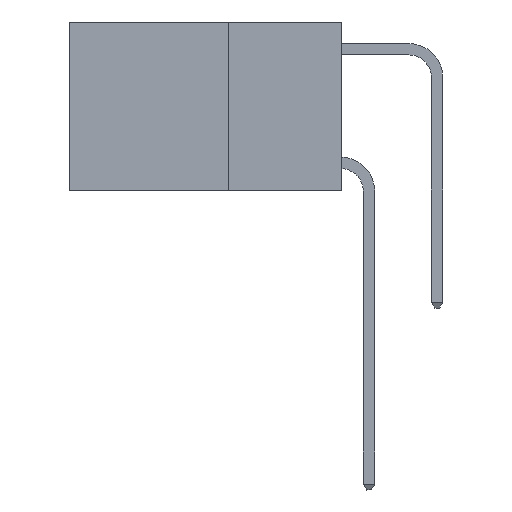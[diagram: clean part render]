
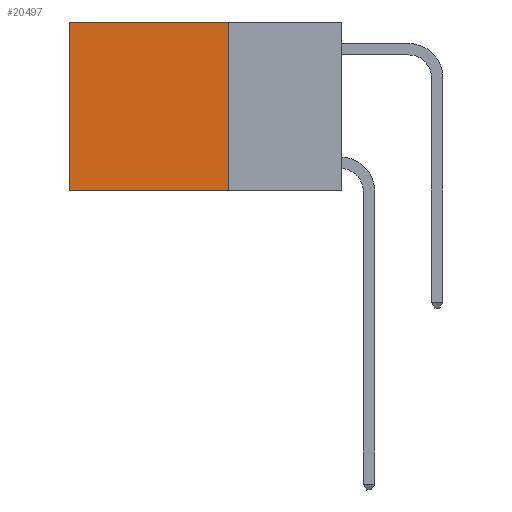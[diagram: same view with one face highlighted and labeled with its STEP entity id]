
A CAD part, left-side view. The second image highlights one B-rep face of the part: STEP entity #20497.
In plain terms, the highlighted planar face has unit normal (-1, 0, 0).
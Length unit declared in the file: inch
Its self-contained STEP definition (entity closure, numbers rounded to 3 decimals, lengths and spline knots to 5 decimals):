
#1419 = CARTESIAN_POINT ( 'NONE',  ( 0.2625, 0.25, -0.37 ) ) ;
#1628 = CARTESIAN_POINT ( 'NONE',  ( 0.2625, 0.25, 0. ) ) ;
#2573 = ORIENTED_EDGE ( 'NONE', *, *, #11147, .T. ) ;
#2826 = VECTOR ( 'NONE', #27915, 39.37008 ) ;
#4253 = DIRECTION ( 'NONE',  ( 0., 0., -1. ) ) ;
#5811 = EDGE_CURVE ( 'NONE', #22602, #11656, #15699, .T. ) ;
#6998 = VECTOR ( 'NONE', #30845, 39.37008 ) ;
#7072 = CARTESIAN_POINT ( 'NONE',  ( 0.2625, 0.6, 0. ) ) ;
#8488 = ORIENTED_EDGE ( 'NONE', *, *, #13996, .F. ) ;
#8857 = LINE ( 'NONE', #1419, #15899 ) ;
#9338 = DIRECTION ( 'NONE',  ( 0., 1., 0. ) ) ;
#10141 = AXIS2_PLACEMENT_3D ( 'NONE', #1628, #20091, #4253 ) ;
#11147 = EDGE_CURVE ( 'NONE', #11656, #28397, #15622, .T. ) ;
#11269 = ORIENTED_EDGE ( 'NONE', *, *, #5811, .T. ) ;
#11656 = VERTEX_POINT ( 'NONE', #7072 ) ;
#13996 = EDGE_CURVE ( 'NONE', #24605, #28397, #8857, .T. ) ;
#14675 = EDGE_LOOP ( 'NONE', ( #2573, #8488, #25299, #11269 ) ) ;
#14751 = PLANE ( 'NONE',  #10141 ) ;
#14977 = CARTESIAN_POINT ( 'NONE',  ( 0.2625, 0.25, -0.37 ) ) ;
#15622 = LINE ( 'NONE', #18229, #21836 ) ;
#15699 = LINE ( 'NONE', #22985, #6998 ) ;
#15899 = VECTOR ( 'NONE', #9338, 39.37008 ) ;
#16224 = FACE_OUTER_BOUND ( 'NONE', #14675, .T. ) ;
#18229 = CARTESIAN_POINT ( 'NONE',  ( 0.2625, 0.6, 0. ) ) ;
#20091 = DIRECTION ( 'NONE',  ( 1., 0., 0. ) ) ;
#20497 = ADVANCED_FACE ( 'NONE', ( #16224 ), #14751, .F. ) ;
#21836 = VECTOR ( 'NONE', #23509, 39.37008 ) ;
#22602 = VERTEX_POINT ( 'NONE', #30933 ) ;
#22985 = CARTESIAN_POINT ( 'NONE',  ( 0.2625, 0.25, 0. ) ) ;
#23509 = DIRECTION ( 'NONE',  ( 0., 0., -1. ) ) ;
#23862 = LINE ( 'NONE', #25297, #2826 ) ;
#24605 = VERTEX_POINT ( 'NONE', #14977 ) ;
#25229 = EDGE_CURVE ( 'NONE', #22602, #24605, #23862, .T. ) ;
#25297 = CARTESIAN_POINT ( 'NONE',  ( 0.2625, 0.25, 0. ) ) ;
#25299 = ORIENTED_EDGE ( 'NONE', *, *, #25229, .F. ) ;
#27915 = DIRECTION ( 'NONE',  ( 0., 0., -1. ) ) ;
#28397 = VERTEX_POINT ( 'NONE', #33039 ) ;
#30845 = DIRECTION ( 'NONE',  ( 0., 1., 0. ) ) ;
#30933 = CARTESIAN_POINT ( 'NONE',  ( 0.2625, 0.25, 0. ) ) ;
#33039 = CARTESIAN_POINT ( 'NONE',  ( 0.2625, 0.6, -0.37 ) ) ;
